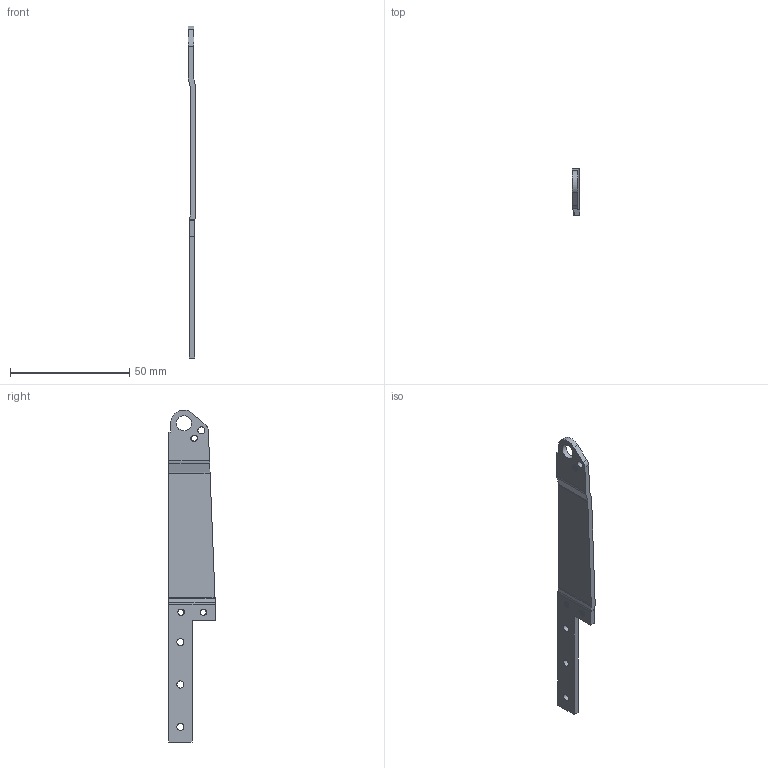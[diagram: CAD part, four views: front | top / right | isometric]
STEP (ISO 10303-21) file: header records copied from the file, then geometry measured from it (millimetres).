
FILE_DESCRIPTION(/* description */ (''),/* implementation_level */ '2;1');
FILE_NAME(/* name */ 'Front SL Side Plate 47.step',/* time_stamp */ '2024-01-16T15:59:29-05:00',/* author */ (''),/* organization */ (''),/* preprocessor_version */ 'ST-DEVELOPER v20',/* originating_system */ 'Autodesk Translation Framework v12.14.0.127',/* authorisation */ '');
FILE_SCHEMA (('AUTOMOTIVE_DESIGN { 1 0 10303 214 3 1 1 }'));
Length unit declared in the file: inch
Products named in the file (1): AR47 Magwell
Bounding box: 3.31 x 19.51 x 139.28 mm (x, y, z)
Volume: 4506.6 mm3; surface area: 4877.3 mm2
Topology: 1 solids, 1 shells, 83 faces, 224 edges, 143 vertices
Faces by surface type: cylinder 48, plane 29, bspline 6
Full cylindrical faces by diameter (mm): 2.529 x3, 3 x4, 3.086 x3, 6.426 x1
Entity records: 4642 total; most frequent: CARTESIAN_POINT 2635, ORIENTED_EDGE 448, DIRECTION 345, EDGE_CURVE 224, VERTEX_POINT 143, AXIS2_PLACEMENT_3D 121, LINE 103, VECTOR 103
